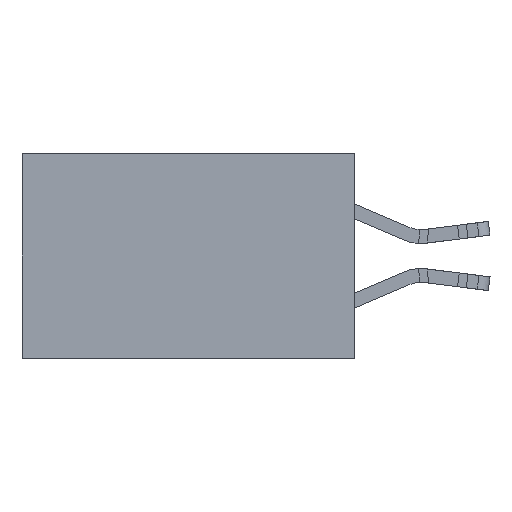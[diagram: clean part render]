
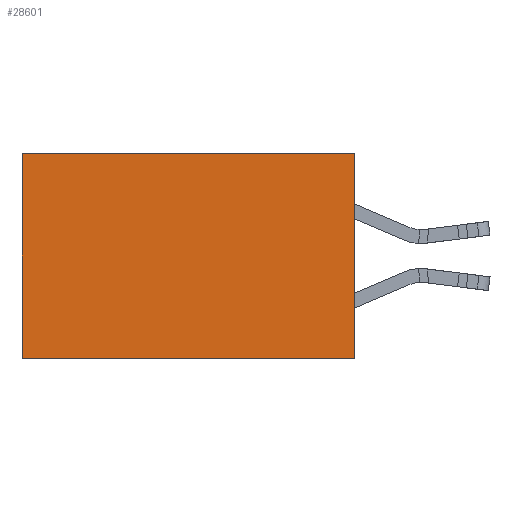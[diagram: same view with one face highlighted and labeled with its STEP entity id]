
A CAD part, left-side view. The second image highlights one B-rep face of the part: STEP entity #28601.
In plain terms, the highlighted planar face has unit normal (-1, 0, 0).
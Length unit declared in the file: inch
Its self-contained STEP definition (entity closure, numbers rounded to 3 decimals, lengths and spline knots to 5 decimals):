
#1384 = VECTOR ( 'NONE', #28617, 39.37008 ) ;
#1920 = CARTESIAN_POINT ( 'NONE',  ( 0.298, 0., 0. ) ) ;
#2310 = CARTESIAN_POINT ( 'NONE',  ( 0.298, 0., -0.37 ) ) ;
#2753 = DIRECTION ( 'NONE',  ( 0., 0., -1. ) ) ;
#7285 = ORIENTED_EDGE ( 'NONE', *, *, #13314, .T. ) ;
#7965 = AXIS2_PLACEMENT_3D ( 'NONE', #18167, #26207, #2753 ) ;
#8204 = LINE ( 'NONE', #13321, #1384 ) ;
#10263 = FACE_OUTER_BOUND ( 'NONE', #27006, .T. ) ;
#11022 = VERTEX_POINT ( 'NONE', #2310 ) ;
#11051 = CARTESIAN_POINT ( 'NONE',  ( 0.298, 0., -0.37 ) ) ;
#12615 = CARTESIAN_POINT ( 'NONE',  ( 0.298, 0.6, -0.37 ) ) ;
#12857 = PLANE ( 'NONE',  #7965 ) ;
#13314 = EDGE_CURVE ( 'NONE', #14542, #31395, #8204, .T. ) ;
#13321 = CARTESIAN_POINT ( 'NONE',  ( 0.298, 0.6, 0. ) ) ;
#13835 = DIRECTION ( 'NONE',  ( 0., 0., -1. ) ) ;
#14274 = LINE ( 'NONE', #29258, #30396 ) ;
#14542 = VERTEX_POINT ( 'NONE', #28918 ) ;
#14668 = LINE ( 'NONE', #1920, #25895 ) ;
#18001 = VECTOR ( 'NONE', #18619, 39.37008 ) ;
#18167 = CARTESIAN_POINT ( 'NONE',  ( 0.298, 0., 0. ) ) ;
#18397 = CARTESIAN_POINT ( 'NONE',  ( 0.298, 0., 0. ) ) ;
#18418 = VERTEX_POINT ( 'NONE', #18397 ) ;
#18446 = ORIENTED_EDGE ( 'NONE', *, *, #21779, .T. ) ;
#18619 = DIRECTION ( 'NONE',  ( 0., 1., 0. ) ) ;
#19371 = ORIENTED_EDGE ( 'NONE', *, *, #30437, .F. ) ;
#21514 = EDGE_CURVE ( 'NONE', #18418, #11022, #14274, .T. ) ;
#21779 = EDGE_CURVE ( 'NONE', #18418, #14542, #14668, .T. ) ;
#22473 = DIRECTION ( 'NONE',  ( 0., 1., 0. ) ) ;
#25895 = VECTOR ( 'NONE', #22473, 39.37008 ) ;
#26207 = DIRECTION ( 'NONE',  ( 1., 0., 0. ) ) ;
#27006 = EDGE_LOOP ( 'NONE', ( #7285, #19371, #29255, #18446 ) ) ;
#28601 = ADVANCED_FACE ( 'NONE', ( #10263 ), #12857, .F. ) ;
#28617 = DIRECTION ( 'NONE',  ( 0., 0., -1. ) ) ;
#28918 = CARTESIAN_POINT ( 'NONE',  ( 0.298, 0.6, 0. ) ) ;
#29255 = ORIENTED_EDGE ( 'NONE', *, *, #21514, .F. ) ;
#29258 = CARTESIAN_POINT ( 'NONE',  ( 0.298, 0., 0. ) ) ;
#30064 = LINE ( 'NONE', #11051, #18001 ) ;
#30396 = VECTOR ( 'NONE', #13835, 39.37008 ) ;
#30437 = EDGE_CURVE ( 'NONE', #11022, #31395, #30064, .T. ) ;
#31395 = VERTEX_POINT ( 'NONE', #12615 ) ;
